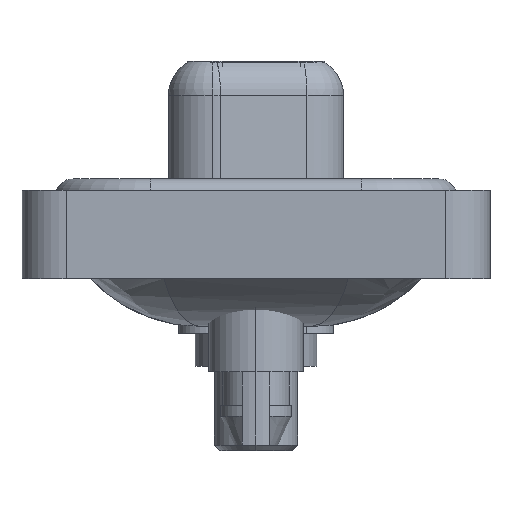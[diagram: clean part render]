
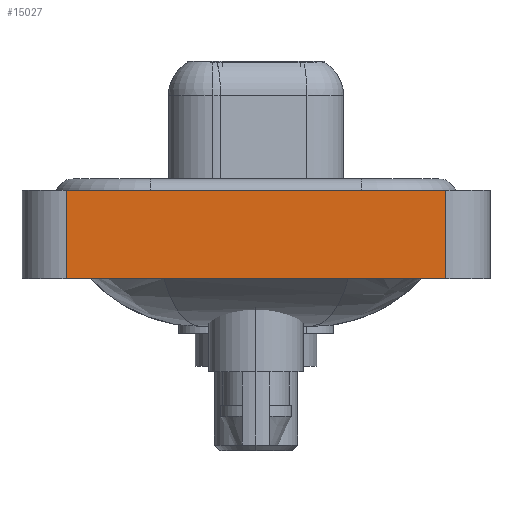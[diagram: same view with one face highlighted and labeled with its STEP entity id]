
A CAD part, left-side view. The second image highlights one B-rep face of the part: STEP entity #15027.
In plain terms, the highlighted planar face has unit normal (-1, 0, 0).
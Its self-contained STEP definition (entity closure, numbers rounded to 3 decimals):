
#219 = ORIENTED_EDGE ( 'NONE', *, *, #7837, .F. ) ;
#616 = VERTEX_POINT ( 'NONE', #15586 ) ;
#694 = VECTOR ( 'NONE', #13777, 1000. ) ;
#3034 = DIRECTION ( 'NONE',  ( 0., 0., 1. ) ) ;
#3077 = CARTESIAN_POINT ( 'NONE',  ( -7.35, -8.55, 0.4 ) ) ;
#3236 = VECTOR ( 'NONE', #6254, 1000. ) ;
#3917 = CARTESIAN_POINT ( 'NONE',  ( -7.35, -8.55, -3.6 ) ) ;
#4149 = CARTESIAN_POINT ( 'NONE',  ( -7.35, -8.55, 0.4 ) ) ;
#4280 = CARTESIAN_POINT ( 'NONE',  ( -7.35, 8.55, 0.4 ) ) ;
#5265 = EDGE_CURVE ( 'NONE', #616, #15904, #15742, .T. ) ;
#5689 = EDGE_LOOP ( 'NONE', ( #16627, #16894, #219, #14825 ) ) ;
#5819 = CARTESIAN_POINT ( 'NONE',  ( -7.35, 8.55, -3.6 ) ) ;
#6212 = FACE_OUTER_BOUND ( 'NONE', #5689, .T. ) ;
#6254 = DIRECTION ( 'NONE',  ( 0., 0., 1. ) ) ;
#7837 = EDGE_CURVE ( 'NONE', #616, #11741, #20922, .T. ) ;
#7965 = AXIS2_PLACEMENT_3D ( 'NONE', #19364, #18034, #3034 ) ;
#10298 = VERTEX_POINT ( 'NONE', #4149 ) ;
#10781 = VECTOR ( 'NONE', #16445, 1000. ) ;
#11471 = CARTESIAN_POINT ( 'NONE',  ( -7.35, -8.55, -3.6 ) ) ;
#11741 = VERTEX_POINT ( 'NONE', #4280 ) ;
#13219 = LINE ( 'NONE', #11471, #18662 ) ;
#13777 = DIRECTION ( 'NONE',  ( 0., -1., 0. ) ) ;
#14825 = ORIENTED_EDGE ( 'NONE', *, *, #5265, .T. ) ;
#15027 = ADVANCED_FACE ( 'NONE', ( #6212 ), #17819, .T. ) ;
#15586 = CARTESIAN_POINT ( 'NONE',  ( -7.35, 8.55, -3.6 ) ) ;
#15742 = LINE ( 'NONE', #3917, #694 ) ;
#15904 = VERTEX_POINT ( 'NONE', #20470 ) ;
#16445 = DIRECTION ( 'NONE',  ( 0., -1., 0. ) ) ;
#16627 = ORIENTED_EDGE ( 'NONE', *, *, #18852, .T. ) ;
#16894 = ORIENTED_EDGE ( 'NONE', *, *, #21581, .F. ) ;
#17819 = PLANE ( 'NONE',  #7965 ) ;
#18034 = DIRECTION ( 'NONE',  ( -1., 0., 0. ) ) ;
#18074 = LINE ( 'NONE', #3077, #10781 ) ;
#18662 = VECTOR ( 'NONE', #21446, 1000. ) ;
#18852 = EDGE_CURVE ( 'NONE', #15904, #10298, #13219, .T. ) ;
#19364 = CARTESIAN_POINT ( 'NONE',  ( -7.35, -8.55, -3.6 ) ) ;
#20470 = CARTESIAN_POINT ( 'NONE',  ( -7.35, -8.55, -3.6 ) ) ;
#20922 = LINE ( 'NONE', #5819, #3236 ) ;
#21446 = DIRECTION ( 'NONE',  ( 0., 0., 1. ) ) ;
#21581 = EDGE_CURVE ( 'NONE', #11741, #10298, #18074, .T. ) ;
